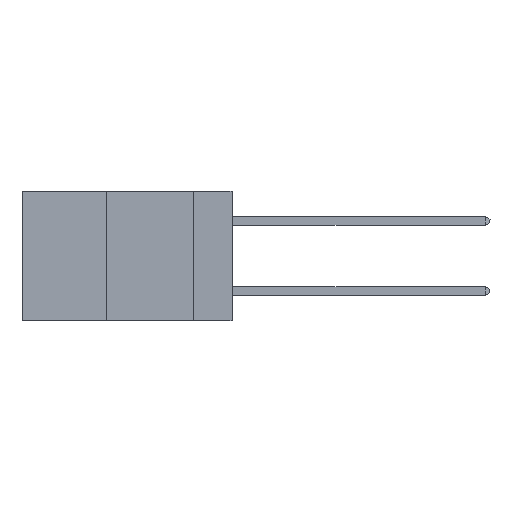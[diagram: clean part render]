
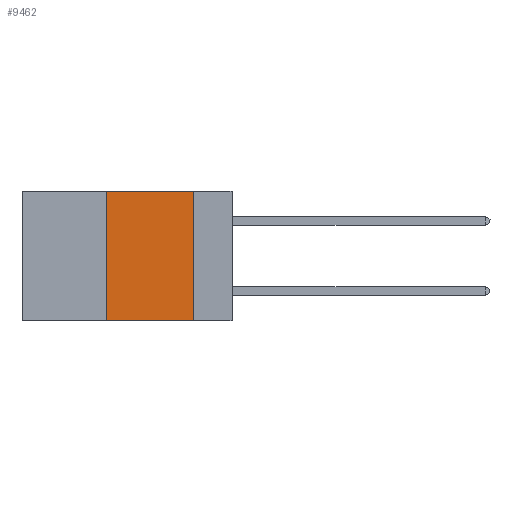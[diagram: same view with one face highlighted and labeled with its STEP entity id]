
A CAD part, left-side view. The second image highlights one B-rep face of the part: STEP entity #9462.
In plain terms, the highlighted planar face has unit normal (-1, 0, 0).
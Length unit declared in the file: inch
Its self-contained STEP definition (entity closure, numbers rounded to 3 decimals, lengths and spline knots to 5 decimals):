
#202 = CARTESIAN_POINT ( 'NONE',  ( 0., 0.36, 0. ) ) ;
#759 = VERTEX_POINT ( 'NONE', #14157 ) ;
#892 = VERTEX_POINT ( 'NONE', #2381 ) ;
#1159 = ORIENTED_EDGE ( 'NONE', *, *, #1712, .T. ) ;
#1712 = EDGE_CURVE ( 'NONE', #759, #20029, #2871, .T. ) ;
#1995 = DIRECTION ( 'NONE',  ( 0., -1., 0. ) ) ;
#2071 = DIRECTION ( 'NONE',  ( 0., 0., 1. ) ) ;
#2297 = VECTOR ( 'NONE', #6159, 39.37008 ) ;
#2381 = CARTESIAN_POINT ( 'NONE',  ( 0., 0.36, 0. ) ) ;
#2575 = CARTESIAN_POINT ( 'NONE',  ( 0., 0.6, -0.37 ) ) ;
#2795 = ORIENTED_EDGE ( 'NONE', *, *, #8959, .F. ) ;
#2871 = LINE ( 'NONE', #2575, #2297 ) ;
#3367 = EDGE_CURVE ( 'NONE', #892, #20063, #10509, .T. ) ;
#3444 = DIRECTION ( 'NONE',  ( 1., 0., 0. ) ) ;
#3804 = VECTOR ( 'NONE', #12043, 39.37008 ) ;
#4273 = CARTESIAN_POINT ( 'NONE',  ( 0., 0.11, -0.37 ) ) ;
#4514 = CARTESIAN_POINT ( 'NONE',  ( 0., 0.11, 0. ) ) ;
#5052 = ORIENTED_EDGE ( 'NONE', *, *, #20229, .F. ) ;
#6159 = DIRECTION ( 'NONE',  ( 0., -1., 0. ) ) ;
#7281 = PLANE ( 'NONE',  #14273 ) ;
#8652 = CARTESIAN_POINT ( 'NONE',  ( 0., 0.11, 0. ) ) ;
#8959 = EDGE_CURVE ( 'NONE', #759, #892, #18728, .T. ) ;
#9462 = ADVANCED_FACE ( 'NONE', ( #17844 ), #7281, .F. ) ;
#10509 = LINE ( 'NONE', #14622, #12518 ) ;
#10672 = LINE ( 'NONE', #8652, #3804 ) ;
#12043 = DIRECTION ( 'NONE',  ( 0., 0., -1. ) ) ;
#12518 = VECTOR ( 'NONE', #1995, 39.37008 ) ;
#13370 = EDGE_LOOP ( 'NONE', ( #5052, #14881, #2795, #1159 ) ) ;
#13912 = VECTOR ( 'NONE', #2071, 39.37008 ) ;
#14157 = CARTESIAN_POINT ( 'NONE',  ( 0., 0.36, -0.37 ) ) ;
#14273 = AXIS2_PLACEMENT_3D ( 'NONE', #23691, #3444, #21945 ) ;
#14622 = CARTESIAN_POINT ( 'NONE',  ( 0., 0.6, 0. ) ) ;
#14881 = ORIENTED_EDGE ( 'NONE', *, *, #3367, .F. ) ;
#17844 = FACE_OUTER_BOUND ( 'NONE', #13370, .T. ) ;
#18728 = LINE ( 'NONE', #202, #13912 ) ;
#20029 = VERTEX_POINT ( 'NONE', #4273 ) ;
#20063 = VERTEX_POINT ( 'NONE', #4514 ) ;
#20229 = EDGE_CURVE ( 'NONE', #20063, #20029, #10672, .T. ) ;
#21945 = DIRECTION ( 'NONE',  ( 0., 0., -1. ) ) ;
#23691 = CARTESIAN_POINT ( 'NONE',  ( 0., 0.6, 0. ) ) ;
